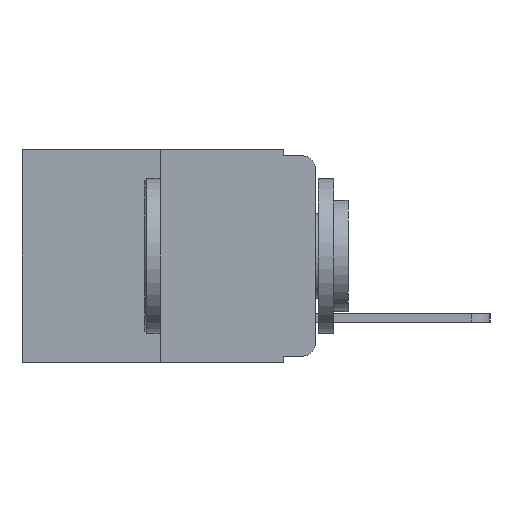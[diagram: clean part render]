
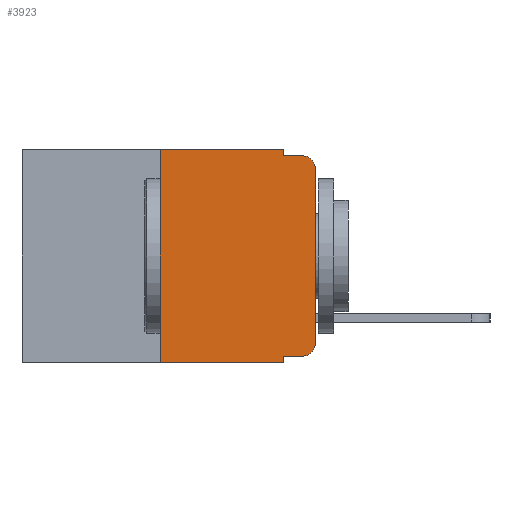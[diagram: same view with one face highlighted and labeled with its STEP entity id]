
A CAD part, left-side view. The second image highlights one B-rep face of the part: STEP entity #3923.
In plain terms, the highlighted planar face has unit normal (-1, 0, 0).
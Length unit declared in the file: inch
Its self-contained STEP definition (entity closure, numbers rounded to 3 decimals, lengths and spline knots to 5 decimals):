
#159 = CARTESIAN_POINT ( 'NONE',  ( 0., 0.25, 0. ) ) ;
#244 = CARTESIAN_POINT ( 'NONE',  ( 0., 0.02, -0.313 ) ) ;
#278 = EDGE_LOOP ( 'NONE', ( #2604, #2841, #6613, #10679, #3709, #2477, #11121, #9601, #6034, #13639 ) ) ;
#692 = VECTOR ( 'NONE', #4488, 39.37008 ) ;
#743 = VECTOR ( 'NONE', #12845, 39.37008 ) ;
#780 = CARTESIAN_POINT ( 'NONE',  ( 0., 0., -0.03 ) ) ;
#936 = DIRECTION ( 'NONE',  ( 0., 0., -1. ) ) ;
#1057 = VERTEX_POINT ( 'NONE', #14119 ) ;
#1617 = DIRECTION ( 'NONE',  ( 0., 0., -1. ) ) ;
#1704 = VERTEX_POINT ( 'NONE', #11942 ) ;
#1742 = LINE ( 'NONE', #7407, #7670 ) ;
#1988 = LINE ( 'NONE', #13063, #10663 ) ;
#2025 = CARTESIAN_POINT ( 'NONE',  ( 0., 0.473, -0.343 ) ) ;
#2070 = CARTESIAN_POINT ( 'NONE',  ( 0., 0.051, 0. ) ) ;
#2137 = DIRECTION ( 'NONE',  ( 0., -1., 0. ) ) ;
#2477 = ORIENTED_EDGE ( 'NONE', *, *, #14780, .F. ) ;
#2604 = ORIENTED_EDGE ( 'NONE', *, *, #3912, .T. ) ;
#2841 = ORIENTED_EDGE ( 'NONE', *, *, #3909, .T. ) ;
#3104 = AXIS2_PLACEMENT_3D ( 'NONE', #10924, #10914, #11491 ) ;
#3403 = EDGE_CURVE ( 'NONE', #8850, #1704, #4119, .T. ) ;
#3709 = ORIENTED_EDGE ( 'NONE', *, *, #4477, .F. ) ;
#3909 = EDGE_CURVE ( 'NONE', #14865, #7095, #5076, .T. ) ;
#3912 = EDGE_CURVE ( 'NONE', #9183, #14865, #1988, .T. ) ;
#3923 = ADVANCED_FACE ( 'NONE', ( #8084 ), #12297, .F. ) ;
#4119 = LINE ( 'NONE', #2025, #6949 ) ;
#4187 = CARTESIAN_POINT ( 'NONE',  ( 0., 0.473, 0. ) ) ;
#4215 = VECTOR ( 'NONE', #936, 39.37008 ) ;
#4477 = EDGE_CURVE ( 'NONE', #12286, #1057, #10346, .T. ) ;
#4488 = DIRECTION ( 'NONE',  ( 0., -1., 0. ) ) ;
#4747 = CARTESIAN_POINT ( 'NONE',  ( 0., 0.051, 0. ) ) ;
#4748 = VERTEX_POINT ( 'NONE', #7617 ) ;
#5033 = CIRCLE ( 'NONE', #8370, 0.02 ) ;
#5076 = CIRCLE ( 'NONE', #3104, 0.02 ) ;
#5137 = CARTESIAN_POINT ( 'NONE',  ( 0., 0.473, 0. ) ) ;
#5689 = AXIS2_PLACEMENT_3D ( 'NONE', #5137, #12327, #10960 ) ;
#5845 = EDGE_CURVE ( 'NONE', #4748, #7095, #1742, .T. ) ;
#5867 = EDGE_CURVE ( 'NONE', #1057, #4748, #7324, .T. ) ;
#5968 = DIRECTION ( 'NONE',  ( 0., 0., 1. ) ) ;
#6021 = DIRECTION ( 'NONE',  ( 0., 0., -1. ) ) ;
#6034 = ORIENTED_EDGE ( 'NONE', *, *, #14598, .T. ) ;
#6277 = CARTESIAN_POINT ( 'NONE',  ( 0., 0.25, -0.343 ) ) ;
#6613 = ORIENTED_EDGE ( 'NONE', *, *, #5845, .F. ) ;
#6770 = CARTESIAN_POINT ( 'NONE',  ( 0., 0., -0.313 ) ) ;
#6949 = VECTOR ( 'NONE', #10423, 39.37008 ) ;
#7095 = VERTEX_POINT ( 'NONE', #11041 ) ;
#7193 = VECTOR ( 'NONE', #6021, 39.37008 ) ;
#7324 = LINE ( 'NONE', #2070, #4215 ) ;
#7407 = CARTESIAN_POINT ( 'NONE',  ( 0., 0.051, -0.01 ) ) ;
#7517 = VERTEX_POINT ( 'NONE', #10501 ) ;
#7617 = CARTESIAN_POINT ( 'NONE',  ( 0., 0.051, -0.01 ) ) ;
#7670 = VECTOR ( 'NONE', #2137, 39.37008 ) ;
#7706 = LINE ( 'NONE', #11199, #692 ) ;
#8084 = FACE_OUTER_BOUND ( 'NONE', #278, .T. ) ;
#8224 = VECTOR ( 'NONE', #5968, 39.37008 ) ;
#8370 = AXIS2_PLACEMENT_3D ( 'NONE', #244, #8875, #1617 ) ;
#8850 = VERTEX_POINT ( 'NONE', #6277 ) ;
#8875 = DIRECTION ( 'NONE',  ( -1., 0., 0. ) ) ;
#9183 = VERTEX_POINT ( 'NONE', #6770 ) ;
#9601 = ORIENTED_EDGE ( 'NONE', *, *, #14859, .F. ) ;
#10346 = LINE ( 'NONE', #4187, #743 ) ;
#10423 = DIRECTION ( 'NONE',  ( 0., -1., 0. ) ) ;
#10462 = LINE ( 'NONE', #4747, #7193 ) ;
#10501 = CARTESIAN_POINT ( 'NONE',  ( 0., 0.02, -0.333 ) ) ;
#10663 = VECTOR ( 'NONE', #12470, 39.37008 ) ;
#10679 = ORIENTED_EDGE ( 'NONE', *, *, #5867, .F. ) ;
#10803 = LINE ( 'NONE', #12479, #8224 ) ;
#10914 = DIRECTION ( 'NONE',  ( -1., 0., 0. ) ) ;
#10924 = CARTESIAN_POINT ( 'NONE',  ( 0., 0.02, -0.03 ) ) ;
#10960 = DIRECTION ( 'NONE',  ( 0., 0., -1. ) ) ;
#11041 = CARTESIAN_POINT ( 'NONE',  ( 0., 0.02, -0.01 ) ) ;
#11121 = ORIENTED_EDGE ( 'NONE', *, *, #3403, .T. ) ;
#11199 = CARTESIAN_POINT ( 'NONE',  ( 0., 0.051, -0.333 ) ) ;
#11491 = DIRECTION ( 'NONE',  ( 0., 0., -1. ) ) ;
#11942 = CARTESIAN_POINT ( 'NONE',  ( 0., 0.051, -0.343 ) ) ;
#12286 = VERTEX_POINT ( 'NONE', #159 ) ;
#12297 = PLANE ( 'NONE',  #5689 ) ;
#12327 = DIRECTION ( 'NONE',  ( 1., 0., 0. ) ) ;
#12470 = DIRECTION ( 'NONE',  ( 0., 0., 1. ) ) ;
#12479 = CARTESIAN_POINT ( 'NONE',  ( 0., 0.25, 0. ) ) ;
#12845 = DIRECTION ( 'NONE',  ( 0., -1., 0. ) ) ;
#13063 = CARTESIAN_POINT ( 'NONE',  ( 0., 0., 0. ) ) ;
#13149 = CARTESIAN_POINT ( 'NONE',  ( 0., 0.051, -0.333 ) ) ;
#13639 = ORIENTED_EDGE ( 'NONE', *, *, #14530, .T. ) ;
#13734 = VERTEX_POINT ( 'NONE', #13149 ) ;
#14119 = CARTESIAN_POINT ( 'NONE',  ( 0., 0.051, 0. ) ) ;
#14530 = EDGE_CURVE ( 'NONE', #7517, #9183, #5033, .T. ) ;
#14598 = EDGE_CURVE ( 'NONE', #13734, #7517, #7706, .T. ) ;
#14780 = EDGE_CURVE ( 'NONE', #8850, #12286, #10803, .T. ) ;
#14859 = EDGE_CURVE ( 'NONE', #13734, #1704, #10462, .T. ) ;
#14865 = VERTEX_POINT ( 'NONE', #780 ) ;
